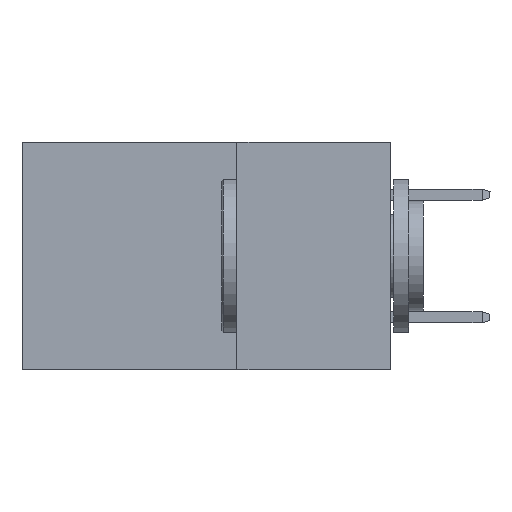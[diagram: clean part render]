
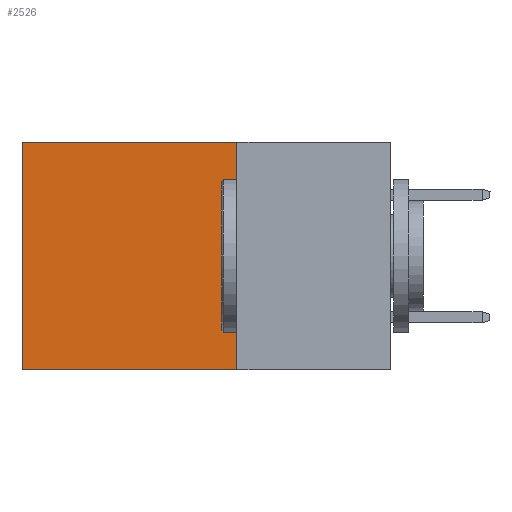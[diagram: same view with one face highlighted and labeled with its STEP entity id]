
A CAD part, left-side view. The second image highlights one B-rep face of the part: STEP entity #2526.
In plain terms, the highlighted planar face has unit normal (-1, 0, 0).
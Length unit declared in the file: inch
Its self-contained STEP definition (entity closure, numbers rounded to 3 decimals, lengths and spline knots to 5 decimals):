
#160 = ORIENTED_EDGE ( 'NONE', *, *, #11419, .T. ) ;
#180 = AXIS2_PLACEMENT_3D ( 'NONE', #2044, #6465, #14090 ) ;
#880 = CARTESIAN_POINT ( 'NONE',  ( 0.2875, 0.6, 0. ) ) ;
#903 = VECTOR ( 'NONE', #8864, 39.37008 ) ;
#1131 = VERTEX_POINT ( 'NONE', #11998 ) ;
#1436 = DIRECTION ( 'NONE',  ( 0., 1., 0. ) ) ;
#2044 = CARTESIAN_POINT ( 'NONE',  ( 0.2875, 0.25, 0. ) ) ;
#2432 = CARTESIAN_POINT ( 'NONE',  ( 0.2875, 0.25, 0. ) ) ;
#2526 = ADVANCED_FACE ( 'NONE', ( #4843 ), #10811, .F. ) ;
#3378 = EDGE_CURVE ( 'NONE', #6187, #4942, #5832, .T. ) ;
#3894 = LINE ( 'NONE', #13210, #903 ) ;
#4051 = ORIENTED_EDGE ( 'NONE', *, *, #3378, .T. ) ;
#4843 = FACE_OUTER_BOUND ( 'NONE', #10240, .T. ) ;
#4942 = VERTEX_POINT ( 'NONE', #880 ) ;
#5505 = VECTOR ( 'NONE', #1436, 39.37008 ) ;
#5832 = LINE ( 'NONE', #9150, #5505 ) ;
#6187 = VERTEX_POINT ( 'NONE', #12757 ) ;
#6465 = DIRECTION ( 'NONE',  ( 1., 0., 0. ) ) ;
#6617 = DIRECTION ( 'NONE',  ( 0., 0., -1. ) ) ;
#7903 = EDGE_CURVE ( 'NONE', #1131, #12270, #3894, .T. ) ;
#8644 = ORIENTED_EDGE ( 'NONE', *, *, #7903, .F. ) ;
#8864 = DIRECTION ( 'NONE',  ( 0., 1., 0. ) ) ;
#9150 = CARTESIAN_POINT ( 'NONE',  ( 0.2875, 0.25, 0. ) ) ;
#9805 = VECTOR ( 'NONE', #11170, 39.37008 ) ;
#10240 = EDGE_LOOP ( 'NONE', ( #160, #8644, #10634, #4051 ) ) ;
#10634 = ORIENTED_EDGE ( 'NONE', *, *, #10897, .F. ) ;
#10811 = PLANE ( 'NONE',  #180 ) ;
#10897 = EDGE_CURVE ( 'NONE', #6187, #1131, #13026, .T. ) ;
#11170 = DIRECTION ( 'NONE',  ( 0., 0., -1. ) ) ;
#11242 = LINE ( 'NONE', #12053, #13807 ) ;
#11419 = EDGE_CURVE ( 'NONE', #4942, #12270, #11242, .T. ) ;
#11998 = CARTESIAN_POINT ( 'NONE',  ( 0.2875, 0.25, -0.37 ) ) ;
#12053 = CARTESIAN_POINT ( 'NONE',  ( 0.2875, 0.6, 0. ) ) ;
#12270 = VERTEX_POINT ( 'NONE', #13664 ) ;
#12757 = CARTESIAN_POINT ( 'NONE',  ( 0.2875, 0.25, 0. ) ) ;
#13026 = LINE ( 'NONE', #2432, #9805 ) ;
#13210 = CARTESIAN_POINT ( 'NONE',  ( 0.2875, 0.25, -0.37 ) ) ;
#13664 = CARTESIAN_POINT ( 'NONE',  ( 0.2875, 0.6, -0.37 ) ) ;
#13807 = VECTOR ( 'NONE', #6617, 39.37008 ) ;
#14090 = DIRECTION ( 'NONE',  ( 0., 0., -1. ) ) ;
